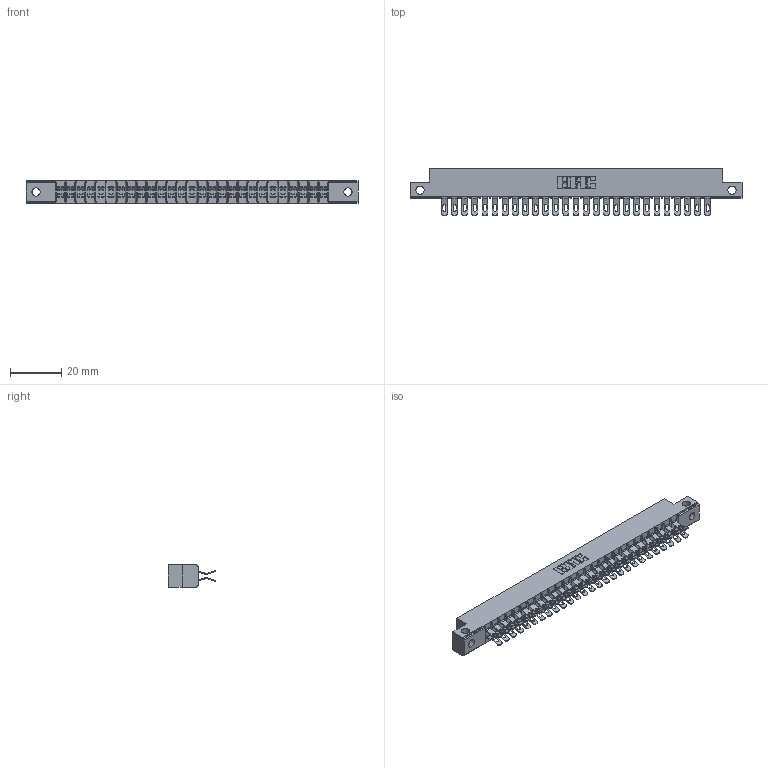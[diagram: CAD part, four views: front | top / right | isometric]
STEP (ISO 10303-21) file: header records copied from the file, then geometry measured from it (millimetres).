
FILE_DESCRIPTION (( 'STEP AP203' ), '1' );
FILE_NAME ('305-054-555-212.STEP', '2020-09-19T23:01:36', ( '' ), ( '' ), 'SwSTEP 2.0', 'SolidWorks 2020', '' );
FILE_SCHEMA (( 'CONFIG_CONTROL_DESIGN' ));
Length unit declared in the file: inch
Products named in the file (3): 305 Part_.128 Dia; 305-054-555-212; 305-290-001_555
Assembly tree (55 placements, depth 2):
  305-054-555-212
    305 Part_.128 Dia
    305-290-001_555  x54
Bounding box: 130 x 18.41 x 8.71 mm (x, y, z)
Volume: 8165.3 mm3; surface area: 16635.4 mm2
Topology: 55 solids, 55 shells, 3692 faces, 11017 edges, 7194 vertices
Faces by surface type: plane 1796, cylinder 1788, sphere 108
Entity records: 32090 total; most frequent: CARTESIAN_POINT 5377, ORIENTED_EDGE 5282, DIRECTION 5147, EDGE_CURVE 2641, VECTOR 2083, LINE 2083, VERTEX_POINT 1682, AXIS2_PLACEMENT_3D 1532
